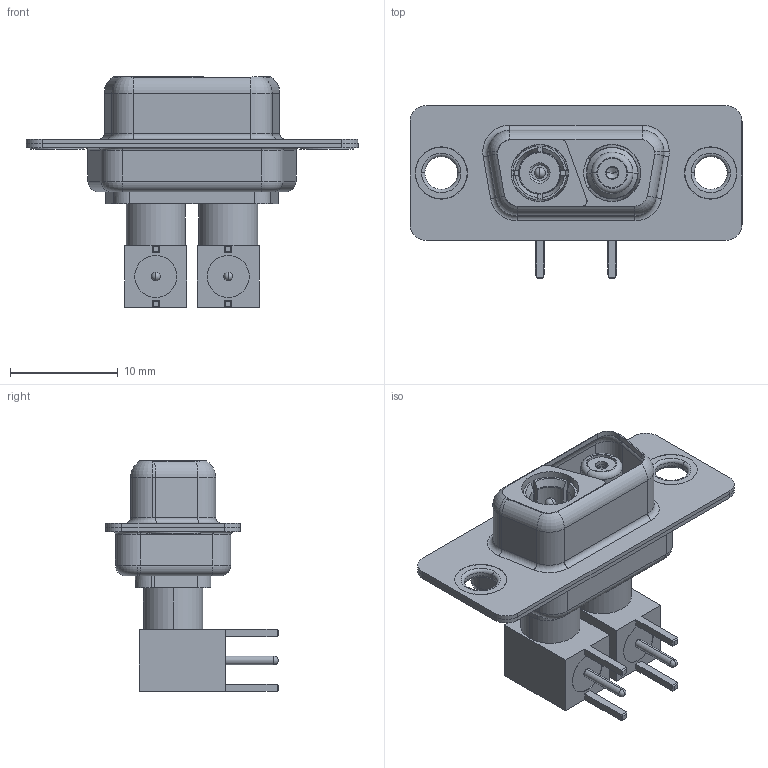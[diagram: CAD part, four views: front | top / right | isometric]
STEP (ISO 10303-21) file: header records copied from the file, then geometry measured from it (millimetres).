
FILE_DESCRIPTION (( 'STEP AP203' ), '1' );
FILE_NAME ('630-2WK2240-5T1.STEP', '2022-05-26T23:20:54', ( '' ), ( '' ), 'SwSTEP 2.0', 'SolidWorks 2020', '' );
FILE_SCHEMA (( 'CONFIG_CONTROL_DESIGN' ));
Length unit declared in the file: millimetre
Products named in the file (17): 630Combo Housing_2WK2; 630-2WK2240-5T1; Co-Ax Jack_RA PC Tail; Co-Ax Jack Assy_RA; Locking Collar; Insulator Socket; Socket_RA; RA Back Shell; Insulator Pin_Straight PC Tail; Pin_RA; 630Combo Shell Front_09 Contacts; Insulator Socket 2; Co-Ax Plug_RA PC Tail; 630Combo Shell Rear_09 Contacts; 630Combo Thru Hole Rivet; Insulator RA Pin; Co-Ax Plug Assy_RA
Assembly tree (20 placements, depth 3):
  630-2WK2240-5T1
    630Combo Housing_2WK2
    630Combo Shell Front_09 Contacts
    630Combo Shell Rear_09 Contacts
    630Combo Thru Hole Rivet  x2
    Co-Ax Plug Assy_RA
      Co-Ax Plug_RA PC Tail
      Insulator Pin_Straight PC Tail
      Pin_RA
      Locking Collar
      RA Back Shell
      Insulator RA Pin
    Co-Ax Jack Assy_RA
      Co-Ax Jack_RA PC Tail
      Insulator Socket
      Insulator Socket 2
      Locking Collar
      Socket_RA
      RA Back Shell
      Insulator RA Pin
Bounding box: 30.8 x 16 x 21.41 mm (x, y, z)
Volume: 1934.1 mm3; surface area: 5422.5 mm2
Topology: 18 solids, 18 shells, 574 faces, 1352 edges, 837 vertices
Faces by surface type: cylinder 254, plane 191, torus 77, cone 44, sphere 6, bspline 2
Entity records: 16603 total; most frequent: CARTESIAN_POINT 2876, DIRECTION 2708, ORIENTED_EDGE 2318, EDGE_CURVE 1159, AXIS2_PLACEMENT_3D 1107, VERTEX_POINT 728, CIRCLE 586, EDGE_LOOP 567
